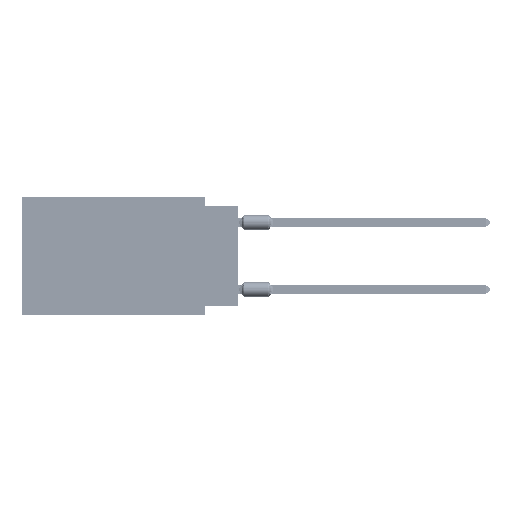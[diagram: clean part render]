
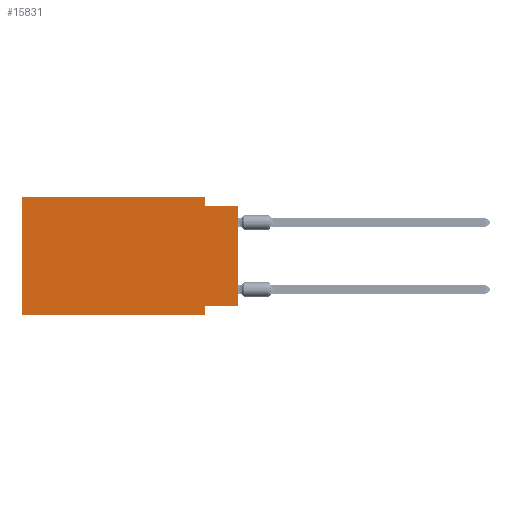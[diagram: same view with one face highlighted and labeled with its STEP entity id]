
A CAD part, left-side view. The second image highlights one B-rep face of the part: STEP entity #15831.
In plain terms, the highlighted planar face has unit normal (-1, 0, 0).
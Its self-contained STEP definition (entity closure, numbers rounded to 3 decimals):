
#3072 = ORIENTED_EDGE ( 'NONE', *, *, #56523, .T. ) ;
#3552 = CARTESIAN_POINT ( 'NONE',  ( 0., 0., -0.635 ) ) ;
#4482 = ORIENTED_EDGE ( 'NONE', *, *, #48110, .F. ) ;
#5567 = EDGE_CURVE ( 'NONE', #52593, #52822, #33912, .T. ) ;
#7766 = VERTEX_POINT ( 'NONE', #36428 ) ;
#8697 = CARTESIAN_POINT ( 'NONE',  ( 0., 0., -8.255 ) ) ;
#9866 = ORIENTED_EDGE ( 'NONE', *, *, #71703, .F. ) ;
#13893 = LINE ( 'NONE', #41272, #79967 ) ;
#15190 = DIRECTION ( 'NONE',  ( 0., 0., 1. ) ) ;
#15831 = ADVANCED_FACE ( 'NONE', ( #63048 ), #98339, .F. ) ;
#17120 = VECTOR ( 'NONE', #96136, 1000. ) ;
#19855 = EDGE_CURVE ( 'NONE', #7766, #54135, #24308, .T. ) ;
#22823 = ORIENTED_EDGE ( 'NONE', *, *, #19855, .F. ) ;
#24308 = LINE ( 'NONE', #117941, #86647 ) ;
#24954 = VECTOR ( 'NONE', #77762, 1000. ) ;
#25362 = CARTESIAN_POINT ( 'NONE',  ( 0., 16.383, 0. ) ) ;
#28581 = CARTESIAN_POINT ( 'NONE',  ( 0., 0., 0. ) ) ;
#29510 = CARTESIAN_POINT ( 'NONE',  ( 0., 16.383, 0. ) ) ;
#30686 = DIRECTION ( 'NONE',  ( 0., -1., 0. ) ) ;
#32797 = ORIENTED_EDGE ( 'NONE', *, *, #5567, .F. ) ;
#33912 = LINE ( 'NONE', #3552, #24954 ) ;
#34473 = DIRECTION ( 'NONE',  ( 1., 0., 0. ) ) ;
#34917 = ORIENTED_EDGE ( 'NONE', *, *, #57729, .T. ) ;
#35061 = CARTESIAN_POINT ( 'NONE',  ( 0., 2.54, -8.255 ) ) ;
#36428 = CARTESIAN_POINT ( 'NONE',  ( 0., 16.383, -8.89 ) ) ;
#37723 = LINE ( 'NONE', #28581, #54494 ) ;
#41272 = CARTESIAN_POINT ( 'NONE',  ( 0., 16.383, -8.89 ) ) ;
#41614 = AXIS2_PLACEMENT_3D ( 'NONE', #25362, #34473, #60655 ) ;
#42563 = EDGE_LOOP ( 'NONE', ( #3072, #32797, #77287, #86051, #22823, #34917, #9866, #4482 ) ) ;
#46377 = DIRECTION ( 'NONE',  ( 0., 0., -1. ) ) ;
#48110 = EDGE_CURVE ( 'NONE', #55995, #53038, #75265, .T. ) ;
#52409 = CARTESIAN_POINT ( 'NONE',  ( 0., 2.54, -0.635 ) ) ;
#52593 = VERTEX_POINT ( 'NONE', #52409 ) ;
#52822 = VERTEX_POINT ( 'NONE', #111352 ) ;
#53038 = VERTEX_POINT ( 'NONE', #35061 ) ;
#54135 = VERTEX_POINT ( 'NONE', #74647 ) ;
#54494 = VECTOR ( 'NONE', #91865, 1000. ) ;
#55995 = VERTEX_POINT ( 'NONE', #8697 ) ;
#56523 = EDGE_CURVE ( 'NONE', #55995, #52822, #37723, .T. ) ;
#57729 = EDGE_CURVE ( 'NONE', #7766, #94085, #13893, .T. ) ;
#57835 = CARTESIAN_POINT ( 'NONE',  ( 0., 2.54, -8.89 ) ) ;
#60014 = CARTESIAN_POINT ( 'NONE',  ( 0., 2.54, 0. ) ) ;
#60655 = DIRECTION ( 'NONE',  ( 0., 0., -1. ) ) ;
#61895 = VECTOR ( 'NONE', #30686, 1000. ) ;
#63048 = FACE_OUTER_BOUND ( 'NONE', #42563, .T. ) ;
#63884 = EDGE_CURVE ( 'NONE', #78846, #52593, #92017, .T. ) ;
#71703 = EDGE_CURVE ( 'NONE', #53038, #94085, #104052, .T. ) ;
#74647 = CARTESIAN_POINT ( 'NONE',  ( 0., 16.383, 0. ) ) ;
#75265 = LINE ( 'NONE', #91119, #94574 ) ;
#77287 = ORIENTED_EDGE ( 'NONE', *, *, #63884, .F. ) ;
#77762 = DIRECTION ( 'NONE',  ( 0., -1., 0. ) ) ;
#78846 = VERTEX_POINT ( 'NONE', #60014 ) ;
#79967 = VECTOR ( 'NONE', #115435, 1000. ) ;
#86051 = ORIENTED_EDGE ( 'NONE', *, *, #112901, .F. ) ;
#86647 = VECTOR ( 'NONE', #15190, 1000. ) ;
#91119 = CARTESIAN_POINT ( 'NONE',  ( 0., 0., -8.255 ) ) ;
#91865 = DIRECTION ( 'NONE',  ( 0., 0., 1. ) ) ;
#92017 = LINE ( 'NONE', #119957, #119581 ) ;
#94085 = VERTEX_POINT ( 'NONE', #117697 ) ;
#94574 = VECTOR ( 'NONE', #102032, 1000. ) ;
#96136 = DIRECTION ( 'NONE',  ( 0., 0., -1. ) ) ;
#98339 = PLANE ( 'NONE',  #41614 ) ;
#102032 = DIRECTION ( 'NONE',  ( 0., 1., 0. ) ) ;
#104052 = LINE ( 'NONE', #57835, #17120 ) ;
#111352 = CARTESIAN_POINT ( 'NONE',  ( 0., 0., -0.635 ) ) ;
#112814 = LINE ( 'NONE', #29510, #61895 ) ;
#112901 = EDGE_CURVE ( 'NONE', #54135, #78846, #112814, .T. ) ;
#115435 = DIRECTION ( 'NONE',  ( 0., -1., 0. ) ) ;
#117697 = CARTESIAN_POINT ( 'NONE',  ( 0., 2.54, -8.89 ) ) ;
#117941 = CARTESIAN_POINT ( 'NONE',  ( 0., 16.383, 0. ) ) ;
#119581 = VECTOR ( 'NONE', #46377, 1000. ) ;
#119957 = CARTESIAN_POINT ( 'NONE',  ( 0., 2.54, 0. ) ) ;
